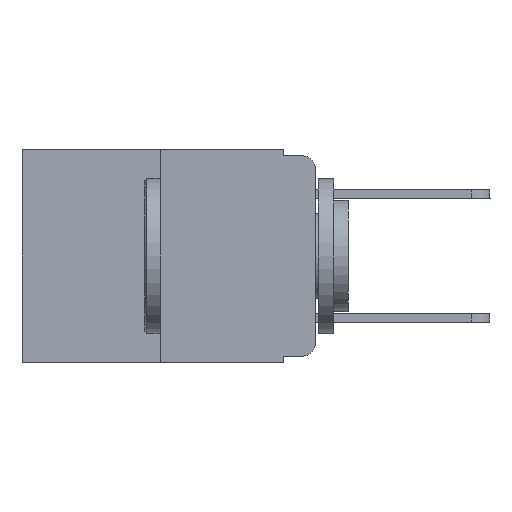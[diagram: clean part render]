
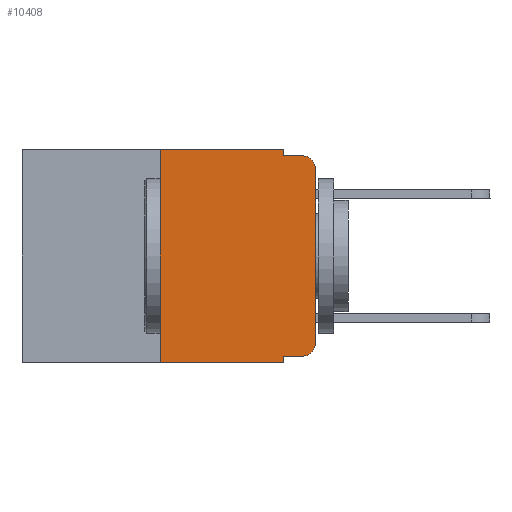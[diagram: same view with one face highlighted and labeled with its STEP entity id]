
A CAD part, left-side view. The second image highlights one B-rep face of the part: STEP entity #10408.
In plain terms, the highlighted planar face has unit normal (-1, 0, 0).
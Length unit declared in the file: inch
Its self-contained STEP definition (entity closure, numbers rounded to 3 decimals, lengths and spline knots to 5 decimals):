
#35 = DIRECTION ( 'NONE',  ( 0., 0., 1. ) ) ;
#151 = VECTOR ( 'NONE', #17471, 39.37008 ) ;
#255 = PLANE ( 'NONE',  #11049 ) ;
#527 = DIRECTION ( 'NONE',  ( 1., 0., 0. ) ) ;
#635 = ORIENTED_EDGE ( 'NONE', *, *, #9657, .F. ) ;
#972 = ORIENTED_EDGE ( 'NONE', *, *, #9659, .F. ) ;
#1288 = LINE ( 'NONE', #8028, #11300 ) ;
#1305 = CARTESIAN_POINT ( 'NONE',  ( 0., 0., -0.03 ) ) ;
#1307 = LINE ( 'NONE', #11029, #6119 ) ;
#1665 = CARTESIAN_POINT ( 'NONE',  ( 0., 0.051, 0. ) ) ;
#2367 = CARTESIAN_POINT ( 'NONE',  ( 0., 0.051, -0.01 ) ) ;
#2435 = AXIS2_PLACEMENT_3D ( 'NONE', #15054, #4072, #9661 ) ;
#2477 = LINE ( 'NONE', #7878, #151 ) ;
#2501 = VERTEX_POINT ( 'NONE', #11184 ) ;
#2572 = CARTESIAN_POINT ( 'NONE',  ( 0., 0.051, -0.333 ) ) ;
#2627 = CARTESIAN_POINT ( 'NONE',  ( 0., 0.02, -0.333 ) ) ;
#2681 = DIRECTION ( 'NONE',  ( 0., -1., 0. ) ) ;
#2729 = VERTEX_POINT ( 'NONE', #5511 ) ;
#2966 = CARTESIAN_POINT ( 'NONE',  ( 0., 0.25, -0.343 ) ) ;
#3216 = DIRECTION ( 'NONE',  ( 0., 0., -1. ) ) ;
#3223 = VERTEX_POINT ( 'NONE', #1305 ) ;
#3610 = ORIENTED_EDGE ( 'NONE', *, *, #12909, .T. ) ;
#3646 = ORIENTED_EDGE ( 'NONE', *, *, #15960, .F. ) ;
#3792 = VERTEX_POINT ( 'NONE', #2627 ) ;
#3854 = EDGE_CURVE ( 'NONE', #3223, #5449, #4555, .T. ) ;
#4023 = CARTESIAN_POINT ( 'NONE',  ( 0., 0.051, -0.343 ) ) ;
#4072 = DIRECTION ( 'NONE',  ( -1., 0., 0. ) ) ;
#4276 = CARTESIAN_POINT ( 'NONE',  ( 0., 0.473, 0. ) ) ;
#4288 = ORIENTED_EDGE ( 'NONE', *, *, #8955, .F. ) ;
#4328 = VECTOR ( 'NONE', #12501, 39.37008 ) ;
#4555 = CIRCLE ( 'NONE', #14609, 0.02 ) ;
#4757 = LINE ( 'NONE', #14567, #7554 ) ;
#4838 = DIRECTION ( 'NONE',  ( 0., 0., 1. ) ) ;
#4995 = LINE ( 'NONE', #17057, #9175 ) ;
#5108 = CARTESIAN_POINT ( 'NONE',  ( 0., 0.051, 0. ) ) ;
#5449 = VERTEX_POINT ( 'NONE', #12712 ) ;
#5457 = VERTEX_POINT ( 'NONE', #16997 ) ;
#5511 = CARTESIAN_POINT ( 'NONE',  ( 0., 0.25, 0. ) ) ;
#6031 = ORIENTED_EDGE ( 'NONE', *, *, #12379, .F. ) ;
#6119 = VECTOR ( 'NONE', #12849, 39.37008 ) ;
#6391 = DIRECTION ( 'NONE',  ( 0., 0., -1. ) ) ;
#7104 = EDGE_CURVE ( 'NONE', #2501, #3792, #15172, .T. ) ;
#7209 = CARTESIAN_POINT ( 'NONE',  ( 0., 0.02, -0.03 ) ) ;
#7554 = VECTOR ( 'NONE', #4838, 39.37008 ) ;
#7878 = CARTESIAN_POINT ( 'NONE',  ( 0., 0.051, -0.01 ) ) ;
#8028 = CARTESIAN_POINT ( 'NONE',  ( 0., 0., 0. ) ) ;
#8428 = VECTOR ( 'NONE', #6391, 39.37008 ) ;
#8655 = ORIENTED_EDGE ( 'NONE', *, *, #9282, .T. ) ;
#8782 = CIRCLE ( 'NONE', #2435, 0.02 ) ;
#8812 = EDGE_LOOP ( 'NONE', ( #8655, #10999, #6031, #3646, #4288, #972, #10457, #635, #12095, #3610 ) ) ;
#8955 = EDGE_CURVE ( 'NONE', #2729, #17581, #1307, .T. ) ;
#9067 = DIRECTION ( 'NONE',  ( 0., 0., -1. ) ) ;
#9175 = VECTOR ( 'NONE', #9067, 39.37008 ) ;
#9282 = EDGE_CURVE ( 'NONE', #5457, #3223, #1288, .T. ) ;
#9657 = EDGE_CURVE ( 'NONE', #2501, #15625, #17092, .T. ) ;
#9659 = EDGE_CURVE ( 'NONE', #9937, #2729, #4757, .T. ) ;
#9661 = DIRECTION ( 'NONE',  ( 0., 0., -1. ) ) ;
#9918 = DIRECTION ( 'NONE',  ( 0., 0., -1. ) ) ;
#9937 = VERTEX_POINT ( 'NONE', #2966 ) ;
#10408 = ADVANCED_FACE ( 'NONE', ( #12509 ), #255, .F. ) ;
#10457 = ORIENTED_EDGE ( 'NONE', *, *, #13870, .T. ) ;
#10999 = ORIENTED_EDGE ( 'NONE', *, *, #3854, .T. ) ;
#11029 = CARTESIAN_POINT ( 'NONE',  ( 0., 0.473, 0. ) ) ;
#11049 = AXIS2_PLACEMENT_3D ( 'NONE', #4276, #527, #3216 ) ;
#11184 = CARTESIAN_POINT ( 'NONE',  ( 0., 0.051, -0.333 ) ) ;
#11300 = VECTOR ( 'NONE', #35, 39.37008 ) ;
#12095 = ORIENTED_EDGE ( 'NONE', *, *, #7104, .T. ) ;
#12379 = EDGE_CURVE ( 'NONE', #16588, #5449, #2477, .T. ) ;
#12501 = DIRECTION ( 'NONE',  ( 0., -1., 0. ) ) ;
#12509 = FACE_OUTER_BOUND ( 'NONE', #8812, .T. ) ;
#12712 = CARTESIAN_POINT ( 'NONE',  ( 0., 0.02, -0.01 ) ) ;
#12849 = DIRECTION ( 'NONE',  ( 0., -1., 0. ) ) ;
#12909 = EDGE_CURVE ( 'NONE', #3792, #5457, #8782, .T. ) ;
#13409 = VECTOR ( 'NONE', #2681, 39.37008 ) ;
#13870 = EDGE_CURVE ( 'NONE', #9937, #15625, #16268, .T. ) ;
#14567 = CARTESIAN_POINT ( 'NONE',  ( 0., 0.25, 0. ) ) ;
#14609 = AXIS2_PLACEMENT_3D ( 'NONE', #7209, #16752, #9918 ) ;
#15054 = CARTESIAN_POINT ( 'NONE',  ( 0., 0.02, -0.313 ) ) ;
#15172 = LINE ( 'NONE', #2572, #4328 ) ;
#15625 = VERTEX_POINT ( 'NONE', #4023 ) ;
#15960 = EDGE_CURVE ( 'NONE', #17581, #16588, #4995, .T. ) ;
#16268 = LINE ( 'NONE', #16449, #13409 ) ;
#16449 = CARTESIAN_POINT ( 'NONE',  ( 0., 0.473, -0.343 ) ) ;
#16588 = VERTEX_POINT ( 'NONE', #2367 ) ;
#16752 = DIRECTION ( 'NONE',  ( -1., 0., 0. ) ) ;
#16997 = CARTESIAN_POINT ( 'NONE',  ( 0., 0., -0.313 ) ) ;
#17057 = CARTESIAN_POINT ( 'NONE',  ( 0., 0.051, 0. ) ) ;
#17092 = LINE ( 'NONE', #5108, #8428 ) ;
#17471 = DIRECTION ( 'NONE',  ( 0., -1., 0. ) ) ;
#17581 = VERTEX_POINT ( 'NONE', #1665 ) ;
